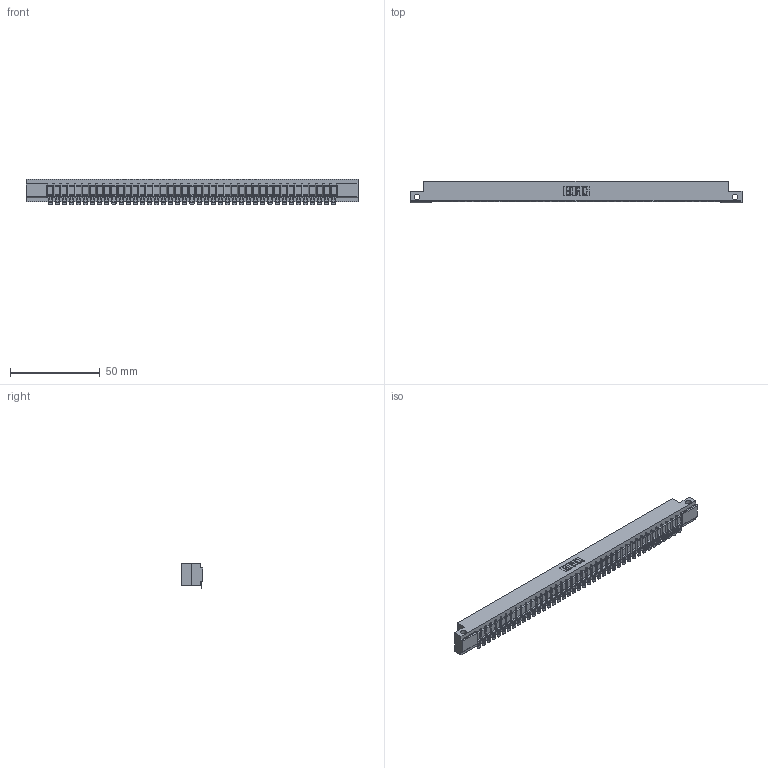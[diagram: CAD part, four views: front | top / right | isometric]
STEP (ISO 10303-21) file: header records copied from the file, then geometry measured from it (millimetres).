
FILE_DESCRIPTION (( 'STEP AP203' ), '1' );
FILE_NAME ('307-041-554-112.STEP', '2019-09-05T11:22:21', ( '' ), ( '' ), 'SwSTEP 2.0', 'SolidWorks 2016', '' );
FILE_SCHEMA (( 'CONFIG_CONTROL_DESIGN' ));
Length unit declared in the file: inch
Products named in the file (3): 307 Part_.128 Dia Side Mounting Holes; 307-290-002_554; 307-041-554-112
Assembly tree (42 placements, depth 2):
  307-041-554-112
    307 Part_.128 Dia Side Mounting Holes
    307-290-002_554  x41
Bounding box: 185.47 x 12.01 x 14.52 mm (x, y, z)
Volume: 19712.9 mm3; surface area: 24911.2 mm2
Topology: 42 solids, 42 shells, 3481 faces, 10696 edges, 7016 vertices
Faces by surface type: plane 1956, cylinder 1441, sphere 84
Entity records: 36239 total; most frequent: CARTESIAN_POINT 6114, ORIENTED_EDGE 6104, DIRECTION 5946, EDGE_CURVE 3052, LINE 2330, VECTOR 2330, VERTEX_POINT 1976, AXIS2_PLACEMENT_3D 1808
